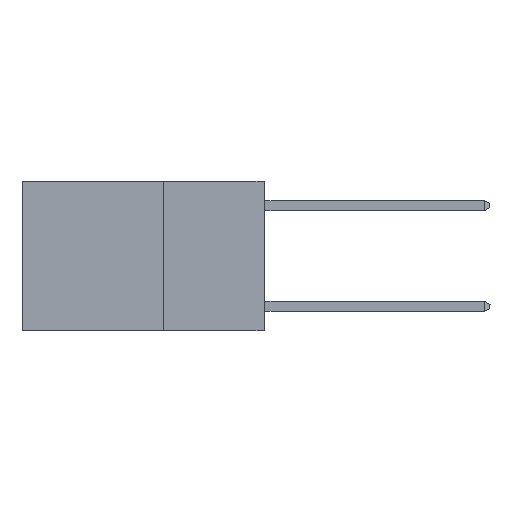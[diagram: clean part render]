
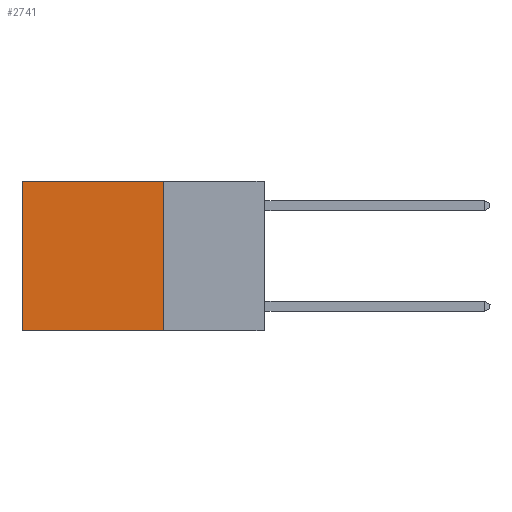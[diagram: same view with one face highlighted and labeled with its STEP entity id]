
A CAD part, left-side view. The second image highlights one B-rep face of the part: STEP entity #2741.
In plain terms, the highlighted planar face has unit normal (-1, 0, 0).
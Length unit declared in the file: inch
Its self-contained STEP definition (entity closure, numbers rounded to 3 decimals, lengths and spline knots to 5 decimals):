
#16 = CARTESIAN_POINT ( 'NONE',  ( 0.2625, 0.25, 0. ) ) ;
#203 = DIRECTION ( 'NONE',  ( 0., 0., -1. ) ) ;
#783 = EDGE_CURVE ( 'NONE', #7092, #11348, #6655, .T. ) ;
#837 = VECTOR ( 'NONE', #203, 39.37008 ) ;
#1166 = EDGE_CURVE ( 'NONE', #9048, #10865, #10922, .T. ) ;
#1609 = PLANE ( 'NONE',  #7196 ) ;
#1656 = DIRECTION ( 'NONE',  ( 1., 0., 0. ) ) ;
#1832 = DIRECTION ( 'NONE',  ( 0., 0., -1. ) ) ;
#2084 = FACE_OUTER_BOUND ( 'NONE', #11624, .T. ) ;
#2550 = EDGE_CURVE ( 'NONE', #10865, #11348, #7615, .T. ) ;
#2741 = ADVANCED_FACE ( 'NONE', ( #2084 ), #1609, .F. ) ;
#2902 = CARTESIAN_POINT ( 'NONE',  ( 0.2625, 0.25, -0.37 ) ) ;
#4252 = DIRECTION ( 'NONE',  ( 0., 0., -1. ) ) ;
#4749 = CARTESIAN_POINT ( 'NONE',  ( 0.2625, 0.25, 0. ) ) ;
#4800 = CARTESIAN_POINT ( 'NONE',  ( 0.2625, 0.25, 0. ) ) ;
#5025 = VECTOR ( 'NONE', #11706, 39.37008 ) ;
#6272 = VECTOR ( 'NONE', #7567, 39.37008 ) ;
#6655 = LINE ( 'NONE', #11370, #837 ) ;
#6772 = CARTESIAN_POINT ( 'NONE',  ( 0.2625, 0.25, -0.37 ) ) ;
#7092 = VERTEX_POINT ( 'NONE', #8645 ) ;
#7196 = AXIS2_PLACEMENT_3D ( 'NONE', #16, #1656, #1832 ) ;
#7567 = DIRECTION ( 'NONE',  ( 0., 1., 0. ) ) ;
#7615 = LINE ( 'NONE', #6772, #5025 ) ;
#8260 = ORIENTED_EDGE ( 'NONE', *, *, #783, .T. ) ;
#8596 = CARTESIAN_POINT ( 'NONE',  ( 0.2625, 0.25, 0. ) ) ;
#8645 = CARTESIAN_POINT ( 'NONE',  ( 0.2625, 0.6, 0. ) ) ;
#8911 = ORIENTED_EDGE ( 'NONE', *, *, #1166, .F. ) ;
#9048 = VERTEX_POINT ( 'NONE', #4749 ) ;
#9188 = LINE ( 'NONE', #8596, #6272 ) ;
#9975 = ORIENTED_EDGE ( 'NONE', *, *, #11308, .T. ) ;
#10865 = VERTEX_POINT ( 'NONE', #2902 ) ;
#10891 = ORIENTED_EDGE ( 'NONE', *, *, #2550, .F. ) ;
#10922 = LINE ( 'NONE', #4800, #11227 ) ;
#11227 = VECTOR ( 'NONE', #4252, 39.37008 ) ;
#11308 = EDGE_CURVE ( 'NONE', #9048, #7092, #9188, .T. ) ;
#11348 = VERTEX_POINT ( 'NONE', #11529 ) ;
#11370 = CARTESIAN_POINT ( 'NONE',  ( 0.2625, 0.6, 0. ) ) ;
#11529 = CARTESIAN_POINT ( 'NONE',  ( 0.2625, 0.6, -0.37 ) ) ;
#11624 = EDGE_LOOP ( 'NONE', ( #8260, #10891, #8911, #9975 ) ) ;
#11706 = DIRECTION ( 'NONE',  ( 0., 1., 0. ) ) ;
